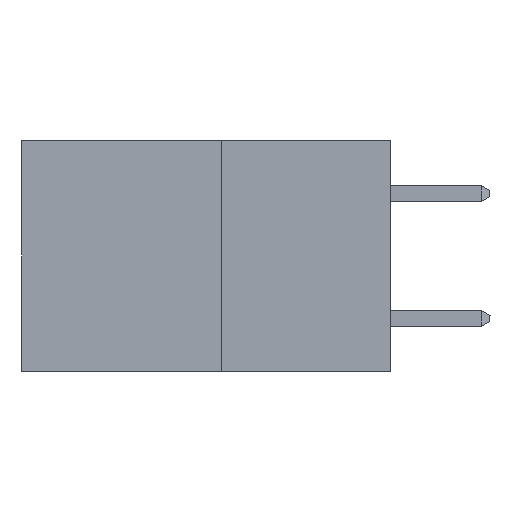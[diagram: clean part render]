
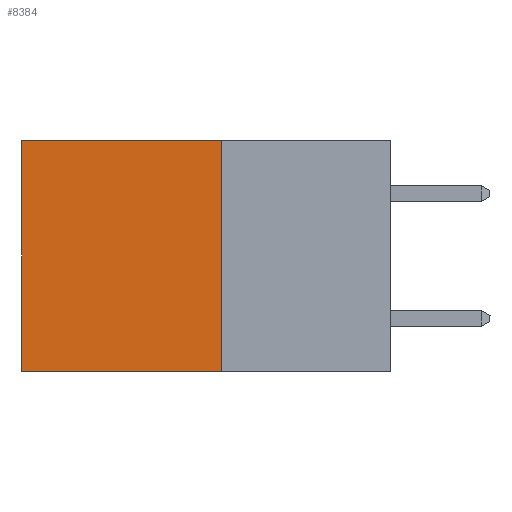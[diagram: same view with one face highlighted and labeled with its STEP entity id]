
A CAD part, left-side view. The second image highlights one B-rep face of the part: STEP entity #8384.
In plain terms, the highlighted planar face has unit normal (-1, 0, 0).
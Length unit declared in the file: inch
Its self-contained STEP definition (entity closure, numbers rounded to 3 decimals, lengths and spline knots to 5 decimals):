
#297 = EDGE_CURVE ( 'NONE', #3164, #6115, #4102, .T. ) ;
#350 = CARTESIAN_POINT ( 'NONE',  ( 0.277, 0.59, 0. ) ) ;
#355 = DIRECTION ( 'NONE',  ( 0., 0., -1. ) ) ;
#1080 = PLANE ( 'NONE',  #4854 ) ;
#1608 = VERTEX_POINT ( 'NONE', #350 ) ;
#1942 = ORIENTED_EDGE ( 'NONE', *, *, #3633, .T. ) ;
#2101 = DIRECTION ( 'NONE',  ( 0., 0., -1. ) ) ;
#2236 = VECTOR ( 'NONE', #6458, 39.37008 ) ;
#2309 = DIRECTION ( 'NONE',  ( 0., 1., 0. ) ) ;
#3128 = EDGE_CURVE ( 'NONE', #3164, #1608, #9505, .T. ) ;
#3164 = VERTEX_POINT ( 'NONE', #9921 ) ;
#3587 = ORIENTED_EDGE ( 'NONE', *, *, #9712, .F. ) ;
#3633 = EDGE_CURVE ( 'NONE', #1608, #6815, #11137, .T. ) ;
#3827 = DIRECTION ( 'NONE',  ( 0., 1., 0. ) ) ;
#3837 = VECTOR ( 'NONE', #355, 39.37008 ) ;
#4102 = LINE ( 'NONE', #4452, #3837 ) ;
#4426 = LINE ( 'NONE', #5018, #5705 ) ;
#4452 = CARTESIAN_POINT ( 'NONE',  ( 0.277, 0.27, -0.37 ) ) ;
#4596 = EDGE_LOOP ( 'NONE', ( #1942, #3587, #8204, #8186 ) ) ;
#4854 = AXIS2_PLACEMENT_3D ( 'NONE', #6560, #7434, #2101 ) ;
#5018 = CARTESIAN_POINT ( 'NONE',  ( 0.277, 0.27, -0.37 ) ) ;
#5705 = VECTOR ( 'NONE', #2309, 39.37008 ) ;
#6115 = VERTEX_POINT ( 'NONE', #7440 ) ;
#6458 = DIRECTION ( 'NONE',  ( 0., 0., -1. ) ) ;
#6560 = CARTESIAN_POINT ( 'NONE',  ( 0.277, 0.27, -0.37 ) ) ;
#6815 = VERTEX_POINT ( 'NONE', #10906 ) ;
#7262 = VECTOR ( 'NONE', #3827, 39.37008 ) ;
#7383 = CARTESIAN_POINT ( 'NONE',  ( 0.277, 0.27, 0. ) ) ;
#7434 = DIRECTION ( 'NONE',  ( 1., 0., 0. ) ) ;
#7440 = CARTESIAN_POINT ( 'NONE',  ( 0.277, 0.27, -0.37 ) ) ;
#8186 = ORIENTED_EDGE ( 'NONE', *, *, #3128, .T. ) ;
#8204 = ORIENTED_EDGE ( 'NONE', *, *, #297, .F. ) ;
#8384 = ADVANCED_FACE ( 'NONE', ( #8975 ), #1080, .F. ) ;
#8975 = FACE_OUTER_BOUND ( 'NONE', #4596, .T. ) ;
#9505 = LINE ( 'NONE', #7383, #7262 ) ;
#9712 = EDGE_CURVE ( 'NONE', #6115, #6815, #4426, .T. ) ;
#9921 = CARTESIAN_POINT ( 'NONE',  ( 0.277, 0.27, 0. ) ) ;
#10614 = CARTESIAN_POINT ( 'NONE',  ( 0.277, 0.59, -0.37 ) ) ;
#10906 = CARTESIAN_POINT ( 'NONE',  ( 0.277, 0.59, -0.37 ) ) ;
#11137 = LINE ( 'NONE', #10614, #2236 ) ;
